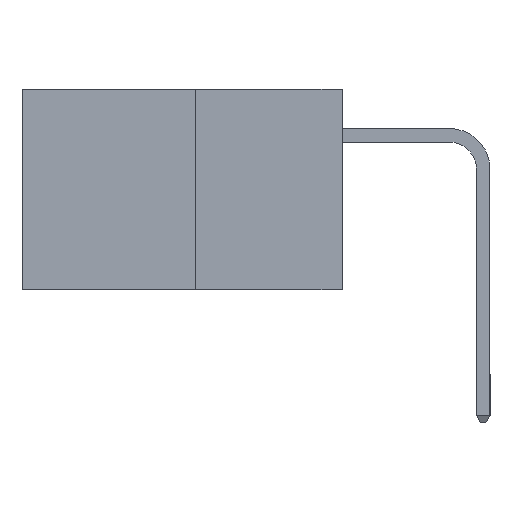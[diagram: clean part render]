
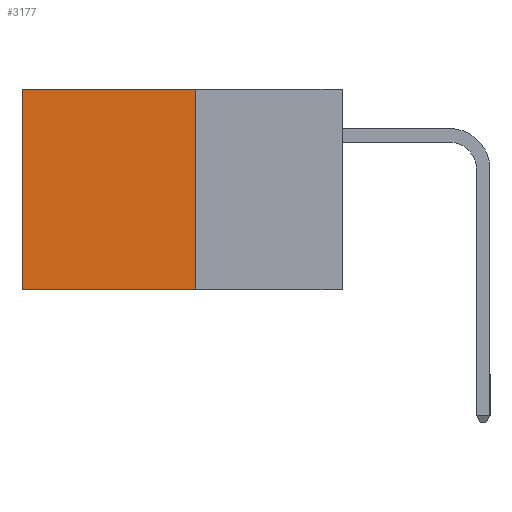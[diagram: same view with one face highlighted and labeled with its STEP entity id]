
A CAD part, left-side view. The second image highlights one B-rep face of the part: STEP entity #3177.
In plain terms, the highlighted planar face has unit normal (-1, 0, 0).
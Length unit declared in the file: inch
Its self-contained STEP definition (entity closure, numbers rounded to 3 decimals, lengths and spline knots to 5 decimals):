
#152 = VECTOR ( 'NONE', #6626, 39.37008 ) ;
#236 = EDGE_CURVE ( 'NONE', #1955, #456, #4876, .T. ) ;
#456 = VERTEX_POINT ( 'NONE', #5305 ) ;
#1955 = VERTEX_POINT ( 'NONE', #6264 ) ;
#2202 = CARTESIAN_POINT ( 'NONE',  ( 0.277, 0.27, -0.37 ) ) ;
#2264 = DIRECTION ( 'NONE',  ( 0., 1., 0. ) ) ;
#2303 = EDGE_CURVE ( 'NONE', #1955, #7075, #2678, .T. ) ;
#2678 = LINE ( 'NONE', #2202, #8503 ) ;
#3145 = ORIENTED_EDGE ( 'NONE', *, *, #3325, .F. ) ;
#3177 = ADVANCED_FACE ( 'NONE', ( #8361 ), #6420, .F. ) ;
#3226 = DIRECTION ( 'NONE',  ( 0., 0., -1. ) ) ;
#3247 = CARTESIAN_POINT ( 'NONE',  ( 0.277, 0.59, -0.37 ) ) ;
#3325 = EDGE_CURVE ( 'NONE', #7075, #6767, #9231, .T. ) ;
#3414 = ORIENTED_EDGE ( 'NONE', *, *, #236, .T. ) ;
#3601 = LINE ( 'NONE', #3247, #7561 ) ;
#4876 = LINE ( 'NONE', #6566, #152 ) ;
#5305 = CARTESIAN_POINT ( 'NONE',  ( 0.277, 0.59, 0. ) ) ;
#5990 = CARTESIAN_POINT ( 'NONE',  ( 0.277, 0.27, -0.37 ) ) ;
#6264 = CARTESIAN_POINT ( 'NONE',  ( 0.277, 0.27, 0. ) ) ;
#6391 = CARTESIAN_POINT ( 'NONE',  ( 0.277, 0.27, -0.37 ) ) ;
#6393 = DIRECTION ( 'NONE',  ( 0., 0., -1. ) ) ;
#6420 = PLANE ( 'NONE',  #7205 ) ;
#6473 = DIRECTION ( 'NONE',  ( 0., 0., -1. ) ) ;
#6566 = CARTESIAN_POINT ( 'NONE',  ( 0.277, 0.27, 0. ) ) ;
#6602 = CARTESIAN_POINT ( 'NONE',  ( 0.277, 0.27, -0.37 ) ) ;
#6626 = DIRECTION ( 'NONE',  ( 0., 1., 0. ) ) ;
#6767 = VERTEX_POINT ( 'NONE', #7433 ) ;
#7075 = VERTEX_POINT ( 'NONE', #5990 ) ;
#7096 = VECTOR ( 'NONE', #2264, 39.37008 ) ;
#7175 = ORIENTED_EDGE ( 'NONE', *, *, #7675, .T. ) ;
#7205 = AXIS2_PLACEMENT_3D ( 'NONE', #6602, #9355, #6393 ) ;
#7402 = ORIENTED_EDGE ( 'NONE', *, *, #2303, .F. ) ;
#7433 = CARTESIAN_POINT ( 'NONE',  ( 0.277, 0.59, -0.37 ) ) ;
#7499 = EDGE_LOOP ( 'NONE', ( #7175, #3145, #7402, #3414 ) ) ;
#7561 = VECTOR ( 'NONE', #3226, 39.37008 ) ;
#7675 = EDGE_CURVE ( 'NONE', #456, #6767, #3601, .T. ) ;
#8361 = FACE_OUTER_BOUND ( 'NONE', #7499, .T. ) ;
#8503 = VECTOR ( 'NONE', #6473, 39.37008 ) ;
#9231 = LINE ( 'NONE', #6391, #7096 ) ;
#9355 = DIRECTION ( 'NONE',  ( 1., 0., 0. ) ) ;
